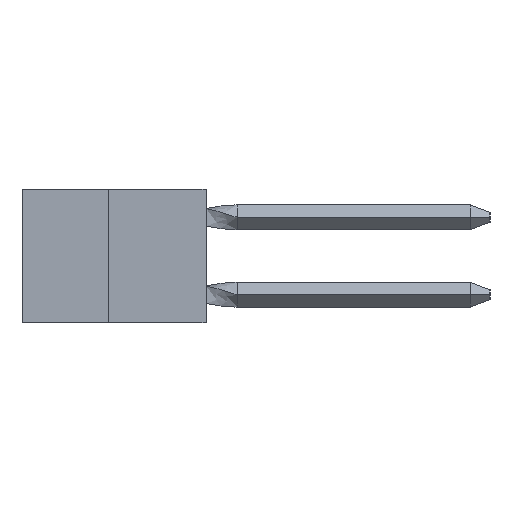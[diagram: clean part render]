
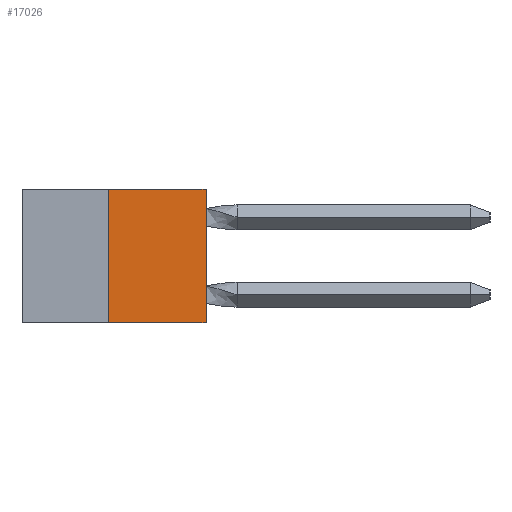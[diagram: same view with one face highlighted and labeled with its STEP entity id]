
A CAD part, left-side view. The second image highlights one B-rep face of the part: STEP entity #17026.
In plain terms, the highlighted planar face has unit normal (-1, 0, 0).
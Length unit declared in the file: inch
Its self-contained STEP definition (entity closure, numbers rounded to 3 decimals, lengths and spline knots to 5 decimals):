
#805 = EDGE_CURVE ( 'NONE', #13207, #38338, #27771, .T. ) ;
#906 = DIRECTION ( 'NONE',  ( 1., 0., 0. ) ) ;
#1717 = DIRECTION ( 'NONE',  ( 0., 0., 1. ) ) ;
#2994 = FACE_OUTER_BOUND ( 'NONE', #33055, .T. ) ;
#4591 = DIRECTION ( 'NONE',  ( 0., -1., 0. ) ) ;
#5068 = LINE ( 'NONE', #43708, #41287 ) ;
#7740 = CARTESIAN_POINT ( 'NONE',  ( 0., 0.473, 0. ) ) ;
#7774 = CARTESIAN_POINT ( 'NONE',  ( 0., 0., 0. ) ) ;
#7856 = AXIS2_PLACEMENT_3D ( 'NONE', #7740, #906, #43444 ) ;
#8044 = CARTESIAN_POINT ( 'NONE',  ( 0., 0.25, 0. ) ) ;
#9262 = LINE ( 'NONE', #7774, #34400 ) ;
#12914 = VERTEX_POINT ( 'NONE', #42055 ) ;
#13207 = VERTEX_POINT ( 'NONE', #29788 ) ;
#14416 = ORIENTED_EDGE ( 'NONE', *, *, #805, .F. ) ;
#14900 = VECTOR ( 'NONE', #26456, 39.37008 ) ;
#14929 = PLANE ( 'NONE',  #7856 ) ;
#17026 = ADVANCED_FACE ( 'NONE', ( #2994 ), #14929, .F. ) ;
#17034 = ORIENTED_EDGE ( 'NONE', *, *, #25839, .T. ) ;
#19386 = VECTOR ( 'NONE', #44557, 39.37008 ) ;
#19805 = CARTESIAN_POINT ( 'NONE',  ( 0., 0.25, 0. ) ) ;
#22364 = CARTESIAN_POINT ( 'NONE',  ( 0., 0., -0.343 ) ) ;
#22547 = EDGE_CURVE ( 'NONE', #13207, #22635, #5068, .T. ) ;
#22635 = VERTEX_POINT ( 'NONE', #22364 ) ;
#25839 = EDGE_CURVE ( 'NONE', #22635, #12914, #9262, .T. ) ;
#26456 = DIRECTION ( 'NONE',  ( 0., -1., 0. ) ) ;
#27771 = LINE ( 'NONE', #19805, #19386 ) ;
#29788 = CARTESIAN_POINT ( 'NONE',  ( 0., 0.25, -0.343 ) ) ;
#30192 = CARTESIAN_POINT ( 'NONE',  ( 0., 0.473, 0. ) ) ;
#33055 = EDGE_LOOP ( 'NONE', ( #40645, #14416, #37358, #17034 ) ) ;
#33908 = LINE ( 'NONE', #30192, #14900 ) ;
#34400 = VECTOR ( 'NONE', #1717, 39.37008 ) ;
#37358 = ORIENTED_EDGE ( 'NONE', *, *, #22547, .T. ) ;
#38338 = VERTEX_POINT ( 'NONE', #8044 ) ;
#38957 = EDGE_CURVE ( 'NONE', #38338, #12914, #33908, .T. ) ;
#40645 = ORIENTED_EDGE ( 'NONE', *, *, #38957, .F. ) ;
#41287 = VECTOR ( 'NONE', #4591, 39.37008 ) ;
#42055 = CARTESIAN_POINT ( 'NONE',  ( 0., 0., 0. ) ) ;
#43444 = DIRECTION ( 'NONE',  ( 0., 0., -1. ) ) ;
#43708 = CARTESIAN_POINT ( 'NONE',  ( 0., 0.473, -0.343 ) ) ;
#44557 = DIRECTION ( 'NONE',  ( 0., 0., 1. ) ) ;
